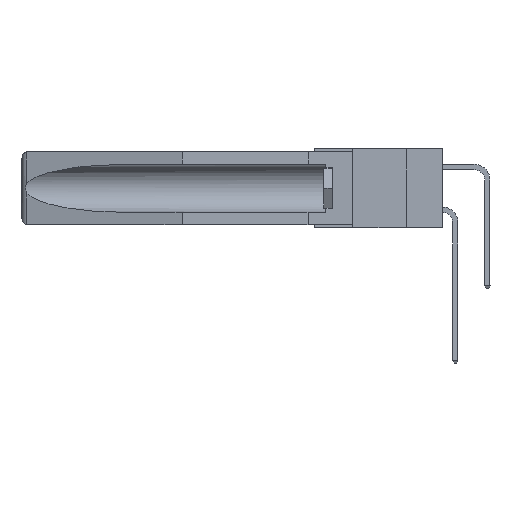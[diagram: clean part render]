
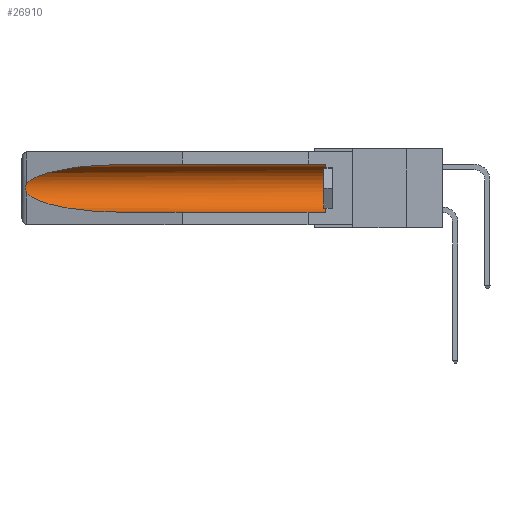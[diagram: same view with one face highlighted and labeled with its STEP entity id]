
A CAD part, left-side view. The second image highlights one B-rep face of the part: STEP entity #26910.
In plain terms, the highlighted cylindrical face has radius 2.857 mm (diameter 5.715 mm), a partial arc.
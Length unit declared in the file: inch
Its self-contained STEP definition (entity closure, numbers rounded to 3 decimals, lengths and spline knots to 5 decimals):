
#39 = ORIENTED_EDGE ( 'NONE', *, *, #3653, .F. ) ;
#707 = DIRECTION ( 'NONE',  ( 0., 1., 0. ) ) ;
#1518 = CARTESIAN_POINT ( 'NONE',  ( 0.26537, 1.52718, -0.14972 ) ) ;
#2482 =( BOUNDED_CURVE ( )  B_SPLINE_CURVE ( 3, ( #24285, #5710, #10289, #5614 ),
 .UNSPECIFIED., .F., .F. ) 
 B_SPLINE_CURVE_WITH_KNOTS ( ( 4, 4 ),
 ( 0.1948, 1.5708 ),
 .UNSPECIFIED. ) 
 CURVE ( )  GEOMETRIC_REPRESENTATION_ITEM ( )  RATIONAL_B_SPLINE_CURVE ( ( 1., 0.848, 0.848, 1. ) ) 
 REPRESENTATION_ITEM ( '' )  );
#2964 = VERTEX_POINT ( 'NONE', #22621 ) ;
#3653 = EDGE_CURVE ( 'NONE', #14003, #29071, #22116, .T. ) ;
#3894 = CIRCLE ( 'NONE', #25438, 0.1125 ) ;
#4360 = AXIS2_PLACEMENT_3D ( 'NONE', #21823, #26487, #24068 ) ;
#4388 = VECTOR ( 'NONE', #27157, 39.37008 ) ;
#5614 = CARTESIAN_POINT ( 'NONE',  ( 0.155, 1.07973, -0.284 ) ) ;
#5710 = CARTESIAN_POINT ( 'NONE',  ( 0.25451, 1.48313, -0.24835 ) ) ;
#6824 = EDGE_LOOP ( 'NONE', ( #19860, #19248, #10472, #39, #28544, #29137 ) ) ;
#7819 = VERTEX_POINT ( 'NONE', #9016 ) ;
#8785 = EDGE_CURVE ( 'NONE', #30074, #7819, #23843, .T. ) ;
#8868 = CARTESIAN_POINT ( 'NONE',  ( 0.2675, 1.53308, -0.17534 ) ) ;
#9016 = CARTESIAN_POINT ( 'NONE',  ( 0.155, 1.07973, -0.059 ) ) ;
#10289 = CARTESIAN_POINT ( 'NONE',  ( 0.21114, 1.30732, -0.284 ) ) ;
#10472 = ORIENTED_EDGE ( 'NONE', *, *, #13068, .T. ) ;
#10717 = EDGE_CURVE ( 'NONE', #14003, #30074, #3894, .T. ) ;
#10856 = CARTESIAN_POINT ( 'NONE',  ( 0.155, -0.30754, -0.059 ) ) ;
#10968 = CARTESIAN_POINT ( 'NONE',  ( 0.155, 0.126, -0.284 ) ) ;
#11063 = DIRECTION ( 'NONE',  ( 0., -1., 0. ) ) ;
#11192 = CARTESIAN_POINT ( 'NONE',  ( 0.155, 1.07973, -0.284 ) ) ;
#12034 = B_SPLINE_CURVE_WITH_KNOTS ( 'NONE', 3,
 ( #1518, #13183, #15902, #18255, #15803, #8868, #20180, #22642, #18050, #20597 ),
 .UNSPECIFIED., .F., .F.,
 ( 4, 2, 2, 2, 4 ),
 ( 0., 0.00029, 0.00058, 0.00087, 0.00117 ),
 .UNSPECIFIED. ) ;
#13068 = EDGE_CURVE ( 'NONE', #2964, #29071, #2482, .T. ) ;
#13183 = CARTESIAN_POINT ( 'NONE',  ( 0.26597, 1.52961, -0.15275 ) ) ;
#14003 = VERTEX_POINT ( 'NONE', #10968 ) ;
#15669 = CARTESIAN_POINT ( 'NONE',  ( 0.21114, 1.30732, -0.059 ) ) ;
#15803 = CARTESIAN_POINT ( 'NONE',  ( 0.2675, 1.53308, -0.16763 ) ) ;
#15902 = CARTESIAN_POINT ( 'NONE',  ( 0.26654, 1.53092, -0.15636 ) ) ;
#16057 = EDGE_CURVE ( 'NONE', #16952, #2964, #12034, .T. ) ;
#16952 = VERTEX_POINT ( 'NONE', #27706 ) ;
#18050 = CARTESIAN_POINT ( 'NONE',  ( 0.26597, 1.5296, -0.19026 ) ) ;
#18255 = CARTESIAN_POINT ( 'NONE',  ( 0.2673, 1.5327, -0.16383 ) ) ;
#18609 = EDGE_CURVE ( 'NONE', #7819, #16952, #25283, .T. ) ;
#19248 = ORIENTED_EDGE ( 'NONE', *, *, #16057, .T. ) ;
#19847 = CYLINDRICAL_SURFACE ( 'NONE', #4360, 0.1125 ) ;
#19860 = ORIENTED_EDGE ( 'NONE', *, *, #18609, .T. ) ;
#20180 = CARTESIAN_POINT ( 'NONE',  ( 0.2673, 1.53269, -0.17917 ) ) ;
#20597 = CARTESIAN_POINT ( 'NONE',  ( 0.26537, 1.52718, -0.19328 ) ) ;
#21823 = CARTESIAN_POINT ( 'NONE',  ( 0.155, -0.30754, -0.1715 ) ) ;
#22116 = LINE ( 'NONE', #24117, #28402 ) ;
#22303 = CARTESIAN_POINT ( 'NONE',  ( 0.155, 0.126, -0.1715 ) ) ;
#22515 = CARTESIAN_POINT ( 'NONE',  ( 0.155, 1.07973, -0.059 ) ) ;
#22621 = CARTESIAN_POINT ( 'NONE',  ( 0.26537, 1.52718, -0.19328 ) ) ;
#22642 = CARTESIAN_POINT ( 'NONE',  ( 0.26655, 1.53094, -0.18657 ) ) ;
#22653 = CARTESIAN_POINT ( 'NONE',  ( 0.155, 0.126, -0.059 ) ) ;
#23843 = LINE ( 'NONE', #10856, #4388 ) ;
#24068 = DIRECTION ( 'NONE',  ( 0., 0., 1. ) ) ;
#24117 = CARTESIAN_POINT ( 'NONE',  ( 0.155, -0.30754, -0.284 ) ) ;
#24285 = CARTESIAN_POINT ( 'NONE',  ( 0.26537, 1.52718, -0.19328 ) ) ;
#25283 =( BOUNDED_CURVE ( )  B_SPLINE_CURVE ( 3, ( #22515, #15669, #27364, #27277 ),
 .UNSPECIFIED., .F., .F. ) 
 B_SPLINE_CURVE_WITH_KNOTS ( ( 4, 4 ),
 ( 4.71239, 6.08839 ),
 .UNSPECIFIED. ) 
 CURVE ( )  GEOMETRIC_REPRESENTATION_ITEM ( )  RATIONAL_B_SPLINE_CURVE ( ( 1., 0.848, 0.848, 1. ) ) 
 REPRESENTATION_ITEM ( '' )  );
#25438 = AXIS2_PLACEMENT_3D ( 'NONE', #22303, #11063, #29166 ) ;
#26487 = DIRECTION ( 'NONE',  ( 0., 1., 0. ) ) ;
#26910 = ADVANCED_FACE ( 'NONE', ( #27600 ), #19847, .F. ) ;
#27157 = DIRECTION ( 'NONE',  ( 0., 1., 0. ) ) ;
#27277 = CARTESIAN_POINT ( 'NONE',  ( 0.26537, 1.52718, -0.14972 ) ) ;
#27364 = CARTESIAN_POINT ( 'NONE',  ( 0.25451, 1.48313, -0.09465 ) ) ;
#27600 = FACE_OUTER_BOUND ( 'NONE', #6824, .T. ) ;
#27706 = CARTESIAN_POINT ( 'NONE',  ( 0.26537, 1.52718, -0.14972 ) ) ;
#28402 = VECTOR ( 'NONE', #707, 39.37008 ) ;
#28544 = ORIENTED_EDGE ( 'NONE', *, *, #10717, .T. ) ;
#29071 = VERTEX_POINT ( 'NONE', #11192 ) ;
#29137 = ORIENTED_EDGE ( 'NONE', *, *, #8785, .T. ) ;
#29166 = DIRECTION ( 'NONE',  ( 0., 0., 1. ) ) ;
#30074 = VERTEX_POINT ( 'NONE', #22653 ) ;
